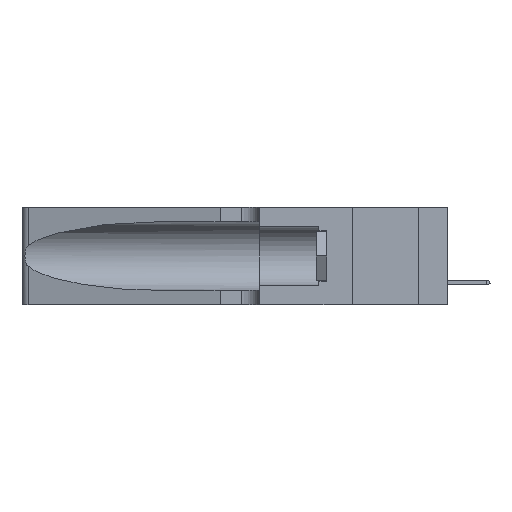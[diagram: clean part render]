
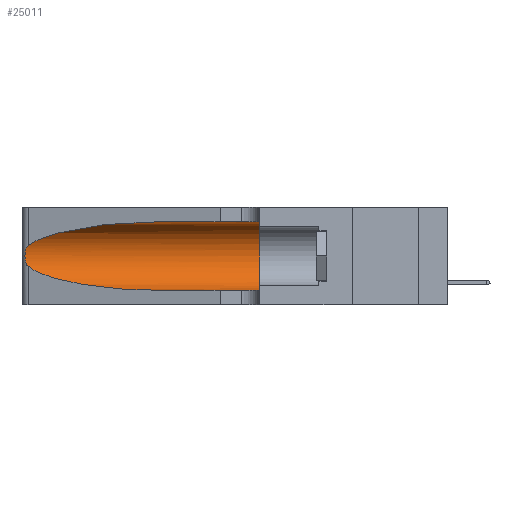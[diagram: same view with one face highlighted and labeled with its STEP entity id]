
A CAD part, left-side view. The second image highlights one B-rep face of the part: STEP entity #25011.
In plain terms, the highlighted cylindrical face has radius 3.308 mm (diameter 6.617 mm), a partial arc.
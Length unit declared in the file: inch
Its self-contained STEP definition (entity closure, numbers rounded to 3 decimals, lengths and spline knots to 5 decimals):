
#353 = CARTESIAN_POINT ( 'NONE',  ( 0.1305, 0.35, 0.05475 ) ) ;
#1543 = CARTESIAN_POINT ( 'NONE',  ( 0.1305, 0.72297, 0.05475 ) ) ;
#2596 = EDGE_CURVE ( 'NONE', #29733, #25225, #26490, .T. ) ;
#2722 = CYLINDRICAL_SURFACE ( 'NONE', #10486, 0.13025 ) ;
#3281 = CARTESIAN_POINT ( 'NONE',  ( 0.26075, 1.23896, 0.178 ) ) ;
#4017 = VERTEX_POINT ( 'NONE', #353 ) ;
#4078 = B_SPLINE_CURVE_WITH_KNOTS ( 'NONE', 3,
 ( #15632, #38076, #34600, #28513, #19221, #15768, #37794, #3281, #19766, #13261, #29322, #6962, #35257, #35531 ),
 .UNSPECIFIED., .F., .F.,
 ( 4, 2, 2, 2, 2, 2, 4 ),
 ( 0., 0.00027, 0.00053, 0.00107, 0.0016, 0.00187, 0.00214 ),
 .UNSPECIFIED. ) ;
#4253 = VECTOR ( 'NONE', #18979, 39.37008 ) ;
#4597 =( BOUNDED_CURVE ( )  B_SPLINE_CURVE ( 3, ( #32993, #39248, #19977, #1543 ),
 .UNSPECIFIED., .F., .T. ) 
 B_SPLINE_CURVE_WITH_KNOTS ( ( 4, 4 ),
 ( 3.44316, 4.71239 ),
 .UNSPECIFIED. ) 
 CURVE ( )  GEOMETRIC_REPRESENTATION_ITEM ( )  RATIONAL_B_SPLINE_CURVE ( ( 1., 0.87, 0.87, 1. ) ) 
 REPRESENTATION_ITEM ( '' )  );
#6675 = DIRECTION ( 'NONE',  ( 0., 0., 1. ) ) ;
#6962 = CARTESIAN_POINT ( 'NONE',  ( 0.25639, 1.23186, 0.15144 ) ) ;
#7531 = CARTESIAN_POINT ( 'NONE',  ( 0.25487, 1.22718, 0.22369 ) ) ;
#7634 = CARTESIAN_POINT ( 'NONE',  ( 0.25487, 1.22718, 0.14631 ) ) ;
#8073 = AXIS2_PLACEMENT_3D ( 'NONE', #11757, #40282, #6675 ) ;
#8147 = ORIENTED_EDGE ( 'NONE', *, *, #34375, .F. ) ;
#8731 = EDGE_CURVE ( 'NONE', #25225, #34014, #4078, .T. ) ;
#9077 = CARTESIAN_POINT ( 'NONE',  ( 0.1305, 0.35, 0.31525 ) ) ;
#10442 = VERTEX_POINT ( 'NONE', #29773 ) ;
#10486 = AXIS2_PLACEMENT_3D ( 'NONE', #39251, #29408, #23129 ) ;
#11259 = LINE ( 'NONE', #20798, #27017 ) ;
#11560 = VERTEX_POINT ( 'NONE', #9077 ) ;
#11757 = CARTESIAN_POINT ( 'NONE',  ( 0.1305, 0.35, 0.185 ) ) ;
#13261 = CARTESIAN_POINT ( 'NONE',  ( 0.25856, 1.23593, 0.16098 ) ) ;
#15632 = CARTESIAN_POINT ( 'NONE',  ( 0.25487, 1.22718, 0.22369 ) ) ;
#15768 = CARTESIAN_POINT ( 'NONE',  ( 0.26018, 1.23835, 0.19895 ) ) ;
#18112 = EDGE_LOOP ( 'NONE', ( #34983, #36802, #23925, #22353, #8147, #40133 ) ) ;
#18979 = DIRECTION ( 'NONE',  ( 0., -1., 0. ) ) ;
#19221 = CARTESIAN_POINT ( 'NONE',  ( 0.25854, 1.2359, 0.20912 ) ) ;
#19766 = CARTESIAN_POINT ( 'NONE',  ( 0.26017, 1.23833, 0.17102 ) ) ;
#19977 = CARTESIAN_POINT ( 'NONE',  ( 0.18966, 0.96281, 0.05475 ) ) ;
#20798 = CARTESIAN_POINT ( 'NONE',  ( 0.1305, 1.61858, 0.05475 ) ) ;
#20896 = FACE_OUTER_BOUND ( 'NONE', #18112, .T. ) ;
#21210 = DIRECTION ( 'NONE',  ( 0., -1., 0. ) ) ;
#21346 = EDGE_CURVE ( 'NONE', #34014, #10442, #4597, .T. ) ;
#22353 = ORIENTED_EDGE ( 'NONE', *, *, #22354, .T. ) ;
#22354 = EDGE_CURVE ( 'NONE', #10442, #4017, #11259, .T. ) ;
#22554 = CARTESIAN_POINT ( 'NONE',  ( 0.1305, 0.72297, 0.31525 ) ) ;
#23129 = DIRECTION ( 'NONE',  ( 0., 0., -1. ) ) ;
#23925 = ORIENTED_EDGE ( 'NONE', *, *, #21346, .T. ) ;
#24416 = EDGE_CURVE ( 'NONE', #29733, #11560, #27817, .T. ) ;
#25011 = ADVANCED_FACE ( 'NONE', ( #20896 ), #2722, .F. ) ;
#25225 = VERTEX_POINT ( 'NONE', #32810 ) ;
#26490 =( BOUNDED_CURVE ( )  B_SPLINE_CURVE ( 3, ( #22554, #30776, #40339, #7531 ),
 .UNSPECIFIED., .F., .T. ) 
 B_SPLINE_CURVE_WITH_KNOTS ( ( 4, 4 ),
 ( 1.5708, 2.84003 ),
 .UNSPECIFIED. ) 
 CURVE ( )  GEOMETRIC_REPRESENTATION_ITEM ( )  RATIONAL_B_SPLINE_CURVE ( ( 1., 0.87, 0.87, 1. ) ) 
 REPRESENTATION_ITEM ( '' )  );
#27017 = VECTOR ( 'NONE', #21210, 39.37008 ) ;
#27817 = LINE ( 'NONE', #34750, #4253 ) ;
#28513 = CARTESIAN_POINT ( 'NONE',  ( 0.25787, 1.23484, 0.2124 ) ) ;
#29322 = CARTESIAN_POINT ( 'NONE',  ( 0.25789, 1.23486, 0.15765 ) ) ;
#29408 = DIRECTION ( 'NONE',  ( 0., -1., 0. ) ) ;
#29733 = VERTEX_POINT ( 'NONE', #39296 ) ;
#29773 = CARTESIAN_POINT ( 'NONE',  ( 0.1305, 0.72297, 0.05475 ) ) ;
#30776 = CARTESIAN_POINT ( 'NONE',  ( 0.18966, 0.96281, 0.31525 ) ) ;
#32810 = CARTESIAN_POINT ( 'NONE',  ( 0.25487, 1.22718, 0.22369 ) ) ;
#32993 = CARTESIAN_POINT ( 'NONE',  ( 0.25487, 1.22718, 0.14631 ) ) ;
#34014 = VERTEX_POINT ( 'NONE', #7634 ) ;
#34375 = EDGE_CURVE ( 'NONE', #11560, #4017, #39892, .T. ) ;
#34600 = CARTESIAN_POINT ( 'NONE',  ( 0.25639, 1.23184, 0.21858 ) ) ;
#34750 = CARTESIAN_POINT ( 'NONE',  ( 0.1305, 1.61858, 0.31525 ) ) ;
#34983 = ORIENTED_EDGE ( 'NONE', *, *, #2596, .T. ) ;
#35257 = CARTESIAN_POINT ( 'NONE',  ( 0.25555, 1.22993, 0.14849 ) ) ;
#35531 = CARTESIAN_POINT ( 'NONE',  ( 0.25487, 1.22718, 0.14631 ) ) ;
#36802 = ORIENTED_EDGE ( 'NONE', *, *, #8731, .T. ) ;
#37794 = CARTESIAN_POINT ( 'NONE',  ( 0.26075, 1.23896, 0.19203 ) ) ;
#38076 = CARTESIAN_POINT ( 'NONE',  ( 0.25555, 1.22994, 0.2215 ) ) ;
#39248 = CARTESIAN_POINT ( 'NONE',  ( 0.2373, 1.15595, 0.08982 ) ) ;
#39251 = CARTESIAN_POINT ( 'NONE',  ( 0.1305, 1.61858, 0.185 ) ) ;
#39296 = CARTESIAN_POINT ( 'NONE',  ( 0.1305, 0.72297, 0.31525 ) ) ;
#39892 = CIRCLE ( 'NONE', #8073, 0.13025 ) ;
#40133 = ORIENTED_EDGE ( 'NONE', *, *, #24416, .F. ) ;
#40282 = DIRECTION ( 'NONE',  ( 0., 1., 0. ) ) ;
#40339 = CARTESIAN_POINT ( 'NONE',  ( 0.2373, 1.15595, 0.28018 ) ) ;
